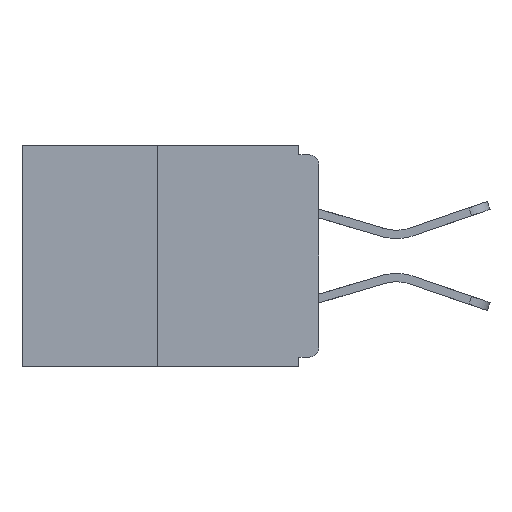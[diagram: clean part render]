
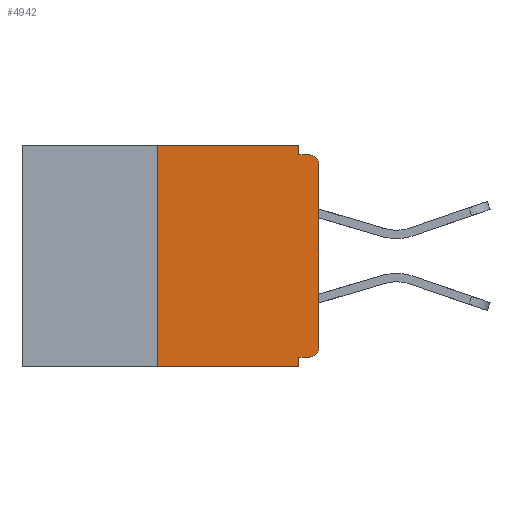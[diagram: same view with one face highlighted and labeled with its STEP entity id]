
A CAD part, left-side view. The second image highlights one B-rep face of the part: STEP entity #4942.
In plain terms, the highlighted planar face has unit normal (-1, 0, 0).
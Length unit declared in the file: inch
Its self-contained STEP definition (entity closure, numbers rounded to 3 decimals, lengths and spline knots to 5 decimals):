
#29 = VERTEX_POINT ( 'NONE', #8220 ) ;
#551 = EDGE_CURVE ( 'NONE', #5381, #5157, #15366, .T. ) ;
#804 = FACE_OUTER_BOUND ( 'NONE', #15424, .T. ) ;
#1155 = VERTEX_POINT ( 'NONE', #18718 ) ;
#1595 = VECTOR ( 'NONE', #24535, 39.37008 ) ;
#1733 = LINE ( 'NONE', #18017, #23942 ) ;
#2558 = CARTESIAN_POINT ( 'NONE',  ( 0., 0.25, -0.343 ) ) ;
#2853 = CARTESIAN_POINT ( 'NONE',  ( 0., 0., -0.328 ) ) ;
#3083 = CARTESIAN_POINT ( 'NONE',  ( 0., 0.46, 0. ) ) ;
#3301 = ORIENTED_EDGE ( 'NONE', *, *, #551, .T. ) ;
#3727 = ORIENTED_EDGE ( 'NONE', *, *, #19663, .F. ) ;
#3787 = EDGE_CURVE ( 'NONE', #11631, #10661, #1733, .T. ) ;
#3993 = ORIENTED_EDGE ( 'NONE', *, *, #14234, .T. ) ;
#4706 = LINE ( 'NONE', #15921, #9291 ) ;
#4942 = ADVANCED_FACE ( 'NONE', ( #804 ), #18907, .F. ) ;
#5157 = VERTEX_POINT ( 'NONE', #13130 ) ;
#5381 = VERTEX_POINT ( 'NONE', #2558 ) ;
#5398 = VECTOR ( 'NONE', #14726, 39.37008 ) ;
#5511 = ORIENTED_EDGE ( 'NONE', *, *, #9703, .F. ) ;
#5546 = LINE ( 'NONE', #18006, #17106 ) ;
#5792 = CARTESIAN_POINT ( 'NONE',  ( 0., 0.031, -0.328 ) ) ;
#6540 = CARTESIAN_POINT ( 'NONE',  ( 0., 0.25, 0. ) ) ;
#6790 = ORIENTED_EDGE ( 'NONE', *, *, #17666, .F. ) ;
#6821 = CARTESIAN_POINT ( 'NONE',  ( 0., 0.25, 0. ) ) ;
#6880 = EDGE_CURVE ( 'NONE', #10133, #29, #24099, .T. ) ;
#7650 = VERTEX_POINT ( 'NONE', #5792 ) ;
#7670 = CIRCLE ( 'NONE', #8034, 0.015 ) ;
#7776 = ORIENTED_EDGE ( 'NONE', *, *, #6880, .T. ) ;
#8034 = AXIS2_PLACEMENT_3D ( 'NONE', #23233, #17398, #21032 ) ;
#8220 = CARTESIAN_POINT ( 'NONE',  ( 0., 0., -0.03 ) ) ;
#8426 = DIRECTION ( 'NONE',  ( 0., 1., 0. ) ) ;
#8574 = EDGE_CURVE ( 'NONE', #7650, #5157, #21499, .T. ) ;
#8898 = CARTESIAN_POINT ( 'NONE',  ( 0., 0.015, -0.015 ) ) ;
#9291 = VECTOR ( 'NONE', #23612, 39.37008 ) ;
#9354 = LINE ( 'NONE', #6821, #5398 ) ;
#9580 = DIRECTION ( 'NONE',  ( 0., 0., -1. ) ) ;
#9703 = EDGE_CURVE ( 'NONE', #13611, #12189, #5546, .T. ) ;
#10057 = ORIENTED_EDGE ( 'NONE', *, *, #8574, .F. ) ;
#10060 = LINE ( 'NONE', #2853, #20990 ) ;
#10109 = DIRECTION ( 'NONE',  ( 0., -1., 0. ) ) ;
#10133 = VERTEX_POINT ( 'NONE', #23093 ) ;
#10650 = AXIS2_PLACEMENT_3D ( 'NONE', #3083, #10773, #16974 ) ;
#10661 = VERTEX_POINT ( 'NONE', #8898 ) ;
#10757 = ORIENTED_EDGE ( 'NONE', *, *, #3787, .F. ) ;
#10773 = DIRECTION ( 'NONE',  ( 1., 0., 0. ) ) ;
#11631 = VERTEX_POINT ( 'NONE', #22231 ) ;
#11709 = CIRCLE ( 'NONE', #18116, 0.015 ) ;
#12189 = VERTEX_POINT ( 'NONE', #21501 ) ;
#12300 = EDGE_CURVE ( 'NONE', #5381, #13611, #9354, .T. ) ;
#12590 = DIRECTION ( 'NONE',  ( -1., 0., 0. ) ) ;
#12719 = ORIENTED_EDGE ( 'NONE', *, *, #18728, .T. ) ;
#13130 = CARTESIAN_POINT ( 'NONE',  ( 0., 0.031, -0.343 ) ) ;
#13611 = VERTEX_POINT ( 'NONE', #6540 ) ;
#14234 = EDGE_CURVE ( 'NONE', #29, #10661, #11709, .T. ) ;
#14436 = DIRECTION ( 'NONE',  ( 0., -1., 0. ) ) ;
#14726 = DIRECTION ( 'NONE',  ( 0., 0., 1. ) ) ;
#15054 = VECTOR ( 'NONE', #10109, 39.37008 ) ;
#15366 = LINE ( 'NONE', #23839, #15054 ) ;
#15424 = EDGE_LOOP ( 'NONE', ( #5511, #18178, #3301, #10057, #3727, #12719, #7776, #3993, #10757, #6790 ) ) ;
#15921 = CARTESIAN_POINT ( 'NONE',  ( 0., 0.031, 0. ) ) ;
#16974 = DIRECTION ( 'NONE',  ( 0., 0., -1. ) ) ;
#17106 = VECTOR ( 'NONE', #17925, 39.37008 ) ;
#17398 = DIRECTION ( 'NONE',  ( -1., 0., 0. ) ) ;
#17666 = EDGE_CURVE ( 'NONE', #12189, #11631, #4706, .T. ) ;
#17925 = DIRECTION ( 'NONE',  ( 0., -1., 0. ) ) ;
#18006 = CARTESIAN_POINT ( 'NONE',  ( 0., 0.46, 0. ) ) ;
#18017 = CARTESIAN_POINT ( 'NONE',  ( 0., 0., -0.015 ) ) ;
#18116 = AXIS2_PLACEMENT_3D ( 'NONE', #18277, #12590, #22516 ) ;
#18178 = ORIENTED_EDGE ( 'NONE', *, *, #12300, .F. ) ;
#18277 = CARTESIAN_POINT ( 'NONE',  ( 0., 0.015, -0.03 ) ) ;
#18524 = CARTESIAN_POINT ( 'NONE',  ( 0., 0., 0. ) ) ;
#18718 = CARTESIAN_POINT ( 'NONE',  ( 0., 0.015, -0.328 ) ) ;
#18728 = EDGE_CURVE ( 'NONE', #1155, #10133, #7670, .T. ) ;
#18907 = PLANE ( 'NONE',  #10650 ) ;
#19663 = EDGE_CURVE ( 'NONE', #1155, #7650, #10060, .T. ) ;
#20990 = VECTOR ( 'NONE', #8426, 39.37008 ) ;
#21032 = DIRECTION ( 'NONE',  ( 0., 0., -1. ) ) ;
#21499 = LINE ( 'NONE', #25031, #22377 ) ;
#21501 = CARTESIAN_POINT ( 'NONE',  ( 0., 0.031, 0. ) ) ;
#22231 = CARTESIAN_POINT ( 'NONE',  ( 0., 0.031, -0.015 ) ) ;
#22377 = VECTOR ( 'NONE', #9580, 39.37008 ) ;
#22516 = DIRECTION ( 'NONE',  ( 0., 0., -1. ) ) ;
#23093 = CARTESIAN_POINT ( 'NONE',  ( 0., 0., -0.313 ) ) ;
#23233 = CARTESIAN_POINT ( 'NONE',  ( 0., 0.015, -0.313 ) ) ;
#23612 = DIRECTION ( 'NONE',  ( 0., 0., -1. ) ) ;
#23839 = CARTESIAN_POINT ( 'NONE',  ( 0., 0.46, -0.343 ) ) ;
#23942 = VECTOR ( 'NONE', #14436, 39.37008 ) ;
#24099 = LINE ( 'NONE', #18524, #1595 ) ;
#24535 = DIRECTION ( 'NONE',  ( 0., 0., 1. ) ) ;
#25031 = CARTESIAN_POINT ( 'NONE',  ( 0., 0.031, -0.343 ) ) ;
